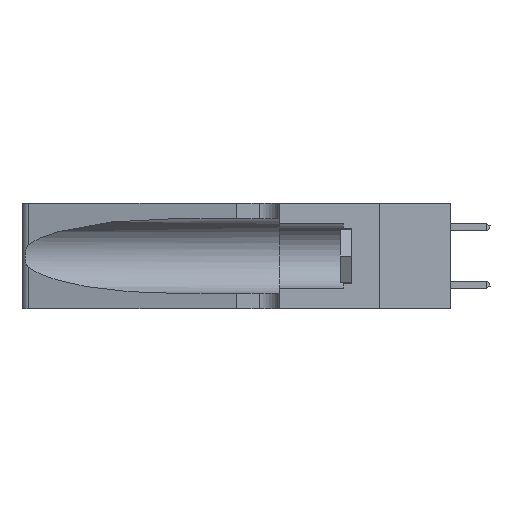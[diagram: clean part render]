
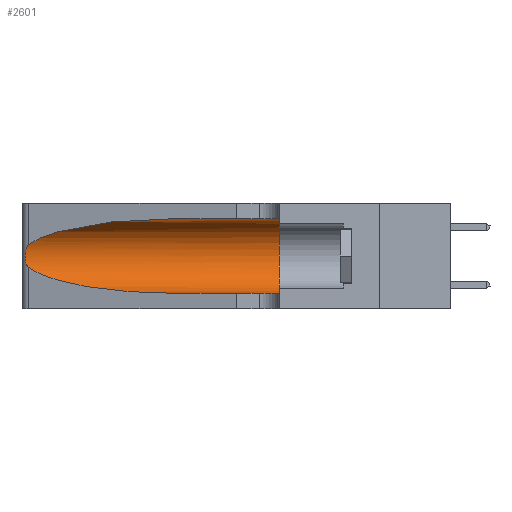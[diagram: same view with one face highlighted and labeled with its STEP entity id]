
A CAD part, left-side view. The second image highlights one B-rep face of the part: STEP entity #2601.
In plain terms, the highlighted cylindrical face has radius 3.308 mm (diameter 6.617 mm), a partial arc.
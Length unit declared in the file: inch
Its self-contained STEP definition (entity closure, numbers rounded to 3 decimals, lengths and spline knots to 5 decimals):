
#395 = VERTEX_POINT ( 'NONE', #1001 ) ;
#452 = CARTESIAN_POINT ( 'NONE',  ( 0.25555, 1.22993, 0.14849 ) ) ;
#1001 = CARTESIAN_POINT ( 'NONE',  ( 0.25487, 1.22718, 0.14631 ) ) ;
#1058 = DIRECTION ( 'NONE',  ( 0., -1., 0. ) ) ;
#1738 = DIRECTION ( 'NONE',  ( 0., -1., 0. ) ) ;
#2146 = LINE ( 'NONE', #22462, #22625 ) ;
#2253 = AXIS2_PLACEMENT_3D ( 'NONE', #19311, #1738, #19044 ) ;
#2601 = ADVANCED_FACE ( 'NONE', ( #17501 ), #22492, .F. ) ;
#2963 = CARTESIAN_POINT ( 'NONE',  ( 0.1305, 0.72297, 0.05475 ) ) ;
#3115 = AXIS2_PLACEMENT_3D ( 'NONE', #24412, #9601, #26856 ) ;
#3437 = CARTESIAN_POINT ( 'NONE',  ( 0.18966, 0.96281, 0.31525 ) ) ;
#3961 = EDGE_CURVE ( 'NONE', #11763, #9164, #11913, .T. ) ;
#4389 = EDGE_CURVE ( 'NONE', #395, #26196, #29085, .T. ) ;
#4536 = CARTESIAN_POINT ( 'NONE',  ( 0.1305, 0.35, 0.05475 ) ) ;
#4601 = ORIENTED_EDGE ( 'NONE', *, *, #3961, .F. ) ;
#4965 = ORIENTED_EDGE ( 'NONE', *, *, #18513, .T. ) ;
#5307 = CARTESIAN_POINT ( 'NONE',  ( 0.25787, 1.23484, 0.2124 ) ) ;
#6988 = EDGE_CURVE ( 'NONE', #26196, #9164, #2146, .T. ) ;
#7774 = CARTESIAN_POINT ( 'NONE',  ( 0.26018, 1.23835, 0.19895 ) ) ;
#8340 = CARTESIAN_POINT ( 'NONE',  ( 0.1305, 0.72297, 0.31525 ) ) ;
#9164 = VERTEX_POINT ( 'NONE', #4536 ) ;
#9601 = DIRECTION ( 'NONE',  ( 0., 1., 0. ) ) ;
#10231 = CARTESIAN_POINT ( 'NONE',  ( 0.26075, 1.23896, 0.178 ) ) ;
#10369 = VERTEX_POINT ( 'NONE', #28725 ) ;
#10735 = EDGE_LOOP ( 'NONE', ( #4965, #18937, #18554, #28511, #4601, #31579 ) ) ;
#10843 = CARTESIAN_POINT ( 'NONE',  ( 0.1305, 1.61858, 0.31525 ) ) ;
#11200 = CARTESIAN_POINT ( 'NONE',  ( 0.25487, 1.22718, 0.14631 ) ) ;
#11763 = VERTEX_POINT ( 'NONE', #26369 ) ;
#11854 =( BOUNDED_CURVE ( )  B_SPLINE_CURVE ( 3, ( #8340, #3437, #30568, #15825 ),
 .UNSPECIFIED., .F., .F. ) 
 B_SPLINE_CURVE_WITH_KNOTS ( ( 4, 4 ),
 ( 1.5708, 2.84003 ),
 .UNSPECIFIED. ) 
 CURVE ( )  GEOMETRIC_REPRESENTATION_ITEM ( )  RATIONAL_B_SPLINE_CURVE ( ( 1., 0.87, 0.87, 1. ) ) 
 REPRESENTATION_ITEM ( '' )  );
#11913 = CIRCLE ( 'NONE', #3115, 0.13025 ) ;
#12733 = CARTESIAN_POINT ( 'NONE',  ( 0.25856, 1.23593, 0.16098 ) ) ;
#13698 = CARTESIAN_POINT ( 'NONE',  ( 0.18966, 0.96281, 0.05475 ) ) ;
#14231 = EDGE_CURVE ( 'NONE', #22365, #11763, #16510, .T. ) ;
#15121 = CARTESIAN_POINT ( 'NONE',  ( 0.25487, 1.22718, 0.22369 ) ) ;
#15233 = CARTESIAN_POINT ( 'NONE',  ( 0.25639, 1.23186, 0.15144 ) ) ;
#15825 = CARTESIAN_POINT ( 'NONE',  ( 0.25487, 1.22718, 0.22369 ) ) ;
#16109 = CARTESIAN_POINT ( 'NONE',  ( 0.2373, 1.15595, 0.08982 ) ) ;
#16510 = LINE ( 'NONE', #10843, #28811 ) ;
#17501 = FACE_OUTER_BOUND ( 'NONE', #10735, .T. ) ;
#17774 = CARTESIAN_POINT ( 'NONE',  ( 0.25487, 1.22718, 0.14631 ) ) ;
#18513 = EDGE_CURVE ( 'NONE', #22365, #10369, #11854, .T. ) ;
#18554 = ORIENTED_EDGE ( 'NONE', *, *, #4389, .T. ) ;
#18937 = ORIENTED_EDGE ( 'NONE', *, *, #24302, .T. ) ;
#19044 = DIRECTION ( 'NONE',  ( 0., 0., -1. ) ) ;
#19311 = CARTESIAN_POINT ( 'NONE',  ( 0.1305, 1.61858, 0.185 ) ) ;
#20125 = CARTESIAN_POINT ( 'NONE',  ( 0.25639, 1.23184, 0.21858 ) ) ;
#20941 = CARTESIAN_POINT ( 'NONE',  ( 0.1305, 0.72297, 0.31525 ) ) ;
#21036 = B_SPLINE_CURVE_WITH_KNOTS ( 'NONE', 3,
 ( #15121, #27395, #20125, #5307, #22591, #7774, #25051, #10231, #27509, #12733, #29983, #15233, #452, #17774 ),
 .UNSPECIFIED., .F., .F.,
 ( 4, 2, 2, 2, 2, 2, 4 ),
 ( 0., 0.00027, 0.00053, 0.00107, 0.0016, 0.00187, 0.00214 ),
 .UNSPECIFIED. ) ;
#22365 = VERTEX_POINT ( 'NONE', #20941 ) ;
#22462 = CARTESIAN_POINT ( 'NONE',  ( 0.1305, 1.61858, 0.05475 ) ) ;
#22492 = CYLINDRICAL_SURFACE ( 'NONE', #2253, 0.13025 ) ;
#22591 = CARTESIAN_POINT ( 'NONE',  ( 0.25854, 1.2359, 0.20912 ) ) ;
#22625 = VECTOR ( 'NONE', #24930, 39.37008 ) ;
#24302 = EDGE_CURVE ( 'NONE', #10369, #395, #21036, .T. ) ;
#24412 = CARTESIAN_POINT ( 'NONE',  ( 0.1305, 0.35, 0.185 ) ) ;
#24930 = DIRECTION ( 'NONE',  ( 0., -1., 0. ) ) ;
#25051 = CARTESIAN_POINT ( 'NONE',  ( 0.26075, 1.23896, 0.19203 ) ) ;
#26196 = VERTEX_POINT ( 'NONE', #2963 ) ;
#26369 = CARTESIAN_POINT ( 'NONE',  ( 0.1305, 0.35, 0.31525 ) ) ;
#26856 = DIRECTION ( 'NONE',  ( 0., 0., 1. ) ) ;
#27395 = CARTESIAN_POINT ( 'NONE',  ( 0.25555, 1.22994, 0.2215 ) ) ;
#27509 = CARTESIAN_POINT ( 'NONE',  ( 0.26017, 1.23833, 0.17102 ) ) ;
#28511 = ORIENTED_EDGE ( 'NONE', *, *, #6988, .T. ) ;
#28725 = CARTESIAN_POINT ( 'NONE',  ( 0.25487, 1.22718, 0.22369 ) ) ;
#28811 = VECTOR ( 'NONE', #1058, 39.37008 ) ;
#29085 =( BOUNDED_CURVE ( )  B_SPLINE_CURVE ( 3, ( #11200, #16109, #13698, #30946 ),
 .UNSPECIFIED., .F., .F. ) 
 B_SPLINE_CURVE_WITH_KNOTS ( ( 4, 4 ),
 ( 3.44316, 4.71239 ),
 .UNSPECIFIED. ) 
 CURVE ( )  GEOMETRIC_REPRESENTATION_ITEM ( )  RATIONAL_B_SPLINE_CURVE ( ( 1., 0.87, 0.87, 1. ) ) 
 REPRESENTATION_ITEM ( '' )  );
#29983 = CARTESIAN_POINT ( 'NONE',  ( 0.25789, 1.23486, 0.15765 ) ) ;
#30568 = CARTESIAN_POINT ( 'NONE',  ( 0.2373, 1.15595, 0.28018 ) ) ;
#30946 = CARTESIAN_POINT ( 'NONE',  ( 0.1305, 0.72297, 0.05475 ) ) ;
#31579 = ORIENTED_EDGE ( 'NONE', *, *, #14231, .F. ) ;
